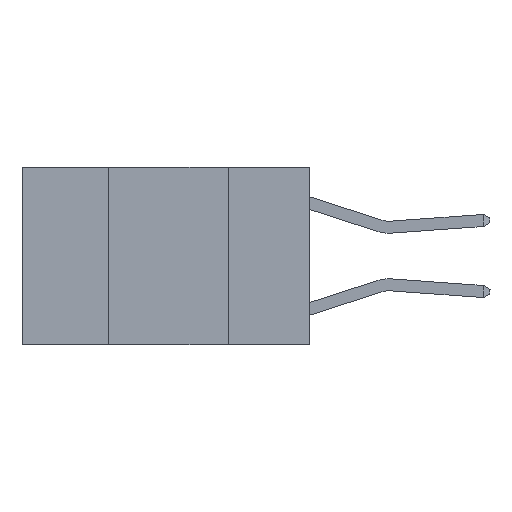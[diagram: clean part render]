
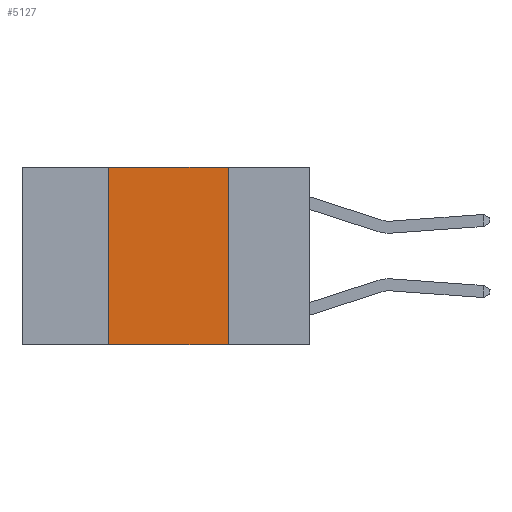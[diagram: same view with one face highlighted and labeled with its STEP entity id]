
A CAD part, left-side view. The second image highlights one B-rep face of the part: STEP entity #5127.
In plain terms, the highlighted planar face has unit normal (-1, 0, 0).
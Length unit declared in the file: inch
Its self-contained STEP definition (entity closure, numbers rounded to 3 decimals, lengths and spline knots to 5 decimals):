
#114 = DIRECTION ( 'NONE',  ( 1., 0., 0. ) ) ;
#473 = AXIS2_PLACEMENT_3D ( 'NONE', #2738, #114, #6961 ) ;
#917 = VECTOR ( 'NONE', #23439, 39.37008 ) ;
#2111 = EDGE_CURVE ( 'NONE', #11501, #21534, #13371, .T. ) ;
#2738 = CARTESIAN_POINT ( 'NONE',  ( 0., 0.6, 0. ) ) ;
#2877 = EDGE_CURVE ( 'NONE', #11716, #21534, #6734, .T. ) ;
#3095 = ORIENTED_EDGE ( 'NONE', *, *, #7327, .F. ) ;
#3180 = VERTEX_POINT ( 'NONE', #3370 ) ;
#3370 = CARTESIAN_POINT ( 'NONE',  ( 0., 0.42, 0. ) ) ;
#5127 = ADVANCED_FACE ( 'NONE', ( #22578 ), #18202, .F. ) ;
#5356 = EDGE_CURVE ( 'NONE', #3180, #11716, #25641, .T. ) ;
#5465 = VECTOR ( 'NONE', #20023, 39.37008 ) ;
#5727 = CARTESIAN_POINT ( 'NONE',  ( 0., 0.17, -0.37 ) ) ;
#6631 = CARTESIAN_POINT ( 'NONE',  ( 0., 0.17, 0. ) ) ;
#6734 = LINE ( 'NONE', #15631, #5465 ) ;
#6961 = DIRECTION ( 'NONE',  ( 0., 0., -1. ) ) ;
#7327 = EDGE_CURVE ( 'NONE', #11501, #3180, #26438, .T. ) ;
#9022 = CARTESIAN_POINT ( 'NONE',  ( 0., 0.6, -0.37 ) ) ;
#10566 = ORIENTED_EDGE ( 'NONE', *, *, #2877, .F. ) ;
#11501 = VERTEX_POINT ( 'NONE', #14090 ) ;
#11716 = VERTEX_POINT ( 'NONE', #6631 ) ;
#13371 = LINE ( 'NONE', #9022, #15622 ) ;
#14090 = CARTESIAN_POINT ( 'NONE',  ( 0., 0.42, -0.37 ) ) ;
#14401 = ORIENTED_EDGE ( 'NONE', *, *, #2111, .T. ) ;
#14526 = CARTESIAN_POINT ( 'NONE',  ( 0., 0.6, 0. ) ) ;
#15622 = VECTOR ( 'NONE', #20233, 39.37008 ) ;
#15631 = CARTESIAN_POINT ( 'NONE',  ( 0., 0.17, 0. ) ) ;
#18202 = PLANE ( 'NONE',  #473 ) ;
#19710 = DIRECTION ( 'NONE',  ( 0., 0., 1. ) ) ;
#19851 = VECTOR ( 'NONE', #19710, 39.37008 ) ;
#20023 = DIRECTION ( 'NONE',  ( 0., 0., -1. ) ) ;
#20233 = DIRECTION ( 'NONE',  ( 0., -1., 0. ) ) ;
#21015 = ORIENTED_EDGE ( 'NONE', *, *, #5356, .F. ) ;
#21534 = VERTEX_POINT ( 'NONE', #5727 ) ;
#22578 = FACE_OUTER_BOUND ( 'NONE', #25351, .T. ) ;
#23439 = DIRECTION ( 'NONE',  ( 0., -1., 0. ) ) ;
#25351 = EDGE_LOOP ( 'NONE', ( #10566, #21015, #3095, #14401 ) ) ;
#25641 = LINE ( 'NONE', #14526, #917 ) ;
#26298 = CARTESIAN_POINT ( 'NONE',  ( 0., 0.42, 0. ) ) ;
#26438 = LINE ( 'NONE', #26298, #19851 ) ;
